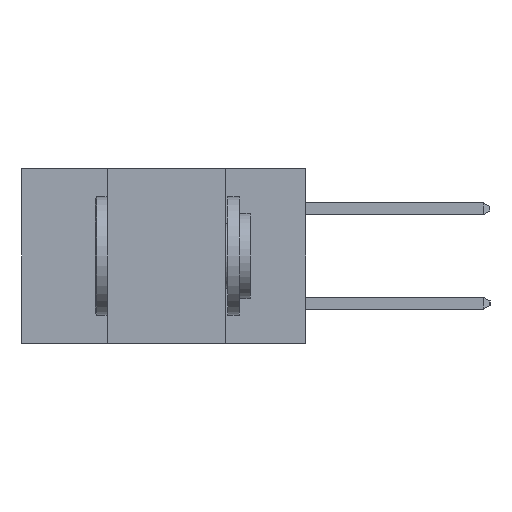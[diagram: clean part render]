
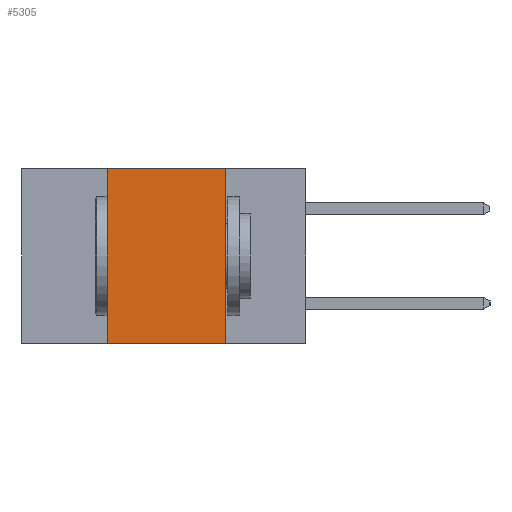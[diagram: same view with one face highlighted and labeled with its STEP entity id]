
A CAD part, left-side view. The second image highlights one B-rep face of the part: STEP entity #5305.
In plain terms, the highlighted planar face has unit normal (-1, 0, 0).
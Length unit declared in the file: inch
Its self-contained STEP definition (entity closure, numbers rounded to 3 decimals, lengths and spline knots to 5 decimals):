
#278 = FACE_OUTER_BOUND ( 'NONE', #7685, .T. ) ;
#713 = VECTOR ( 'NONE', #11557, 39.37008 ) ;
#1255 = VERTEX_POINT ( 'NONE', #2262 ) ;
#1337 = ORIENTED_EDGE ( 'NONE', *, *, #3723, .T. ) ;
#2040 = ORIENTED_EDGE ( 'NONE', *, *, #8685, .F. ) ;
#2068 = ORIENTED_EDGE ( 'NONE', *, *, #5775, .F. ) ;
#2262 = CARTESIAN_POINT ( 'NONE',  ( 0., 0.17, -0.37 ) ) ;
#3723 = EDGE_CURVE ( 'NONE', #4577, #1255, #9934, .T. ) ;
#3931 = ORIENTED_EDGE ( 'NONE', *, *, #9332, .F. ) ;
#4507 = DIRECTION ( 'NONE',  ( 0., 0., -1. ) ) ;
#4577 = VERTEX_POINT ( 'NONE', #5796 ) ;
#4735 = CARTESIAN_POINT ( 'NONE',  ( 0., 0.17, -0.37 ) ) ;
#5286 = VERTEX_POINT ( 'NONE', #10743 ) ;
#5305 = ADVANCED_FACE ( 'NONE', ( #278 ), #6934, .F. ) ;
#5775 = EDGE_CURVE ( 'NONE', #4577, #5286, #10792, .T. ) ;
#5778 = AXIS2_PLACEMENT_3D ( 'NONE', #10799, #10666, #10647 ) ;
#5796 = CARTESIAN_POINT ( 'NONE',  ( 0., 0.42, -0.37 ) ) ;
#6934 = PLANE ( 'NONE',  #5778 ) ;
#7685 = EDGE_LOOP ( 'NONE', ( #3931, #2040, #2068, #1337 ) ) ;
#7847 = VECTOR ( 'NONE', #7905, 39.37008 ) ;
#7905 = DIRECTION ( 'NONE',  ( 0., 0., 1. ) ) ;
#8069 = CARTESIAN_POINT ( 'NONE',  ( 0., 0.42, -0.37 ) ) ;
#8586 = LINE ( 'NONE', #10738, #713 ) ;
#8685 = EDGE_CURVE ( 'NONE', #5286, #10818, #8586, .T. ) ;
#9041 = LINE ( 'NONE', #4735, #11272 ) ;
#9332 = EDGE_CURVE ( 'NONE', #10818, #1255, #9041, .T. ) ;
#9823 = CARTESIAN_POINT ( 'NONE',  ( 0., 0.17, 0. ) ) ;
#9934 = LINE ( 'NONE', #10025, #12670 ) ;
#10025 = CARTESIAN_POINT ( 'NONE',  ( 0., 0.6, -0.37 ) ) ;
#10452 = DIRECTION ( 'NONE',  ( 0., -1., 0. ) ) ;
#10647 = DIRECTION ( 'NONE',  ( 0., 0., -1. ) ) ;
#10666 = DIRECTION ( 'NONE',  ( 1., 0., 0. ) ) ;
#10738 = CARTESIAN_POINT ( 'NONE',  ( 0., 0.6, 0. ) ) ;
#10743 = CARTESIAN_POINT ( 'NONE',  ( 0., 0.42, 0. ) ) ;
#10792 = LINE ( 'NONE', #8069, #7847 ) ;
#10799 = CARTESIAN_POINT ( 'NONE',  ( 0., 0.6, 0. ) ) ;
#10818 = VERTEX_POINT ( 'NONE', #9823 ) ;
#11272 = VECTOR ( 'NONE', #4507, 39.37008 ) ;
#11557 = DIRECTION ( 'NONE',  ( 0., -1., 0. ) ) ;
#12670 = VECTOR ( 'NONE', #10452, 39.37008 ) ;
